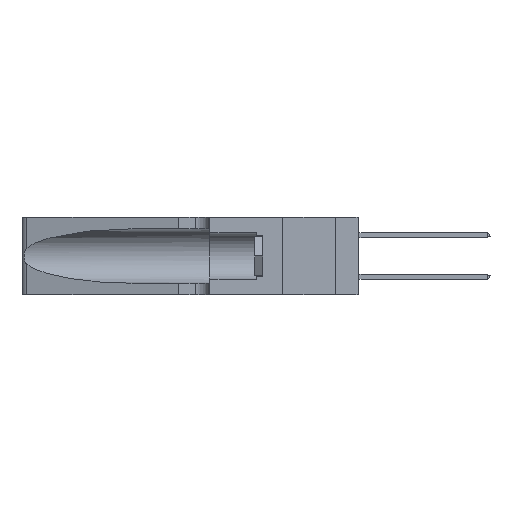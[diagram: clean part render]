
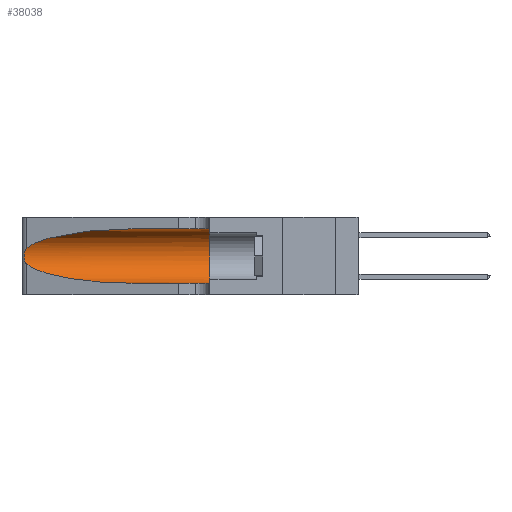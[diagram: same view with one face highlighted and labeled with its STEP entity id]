
A CAD part, left-side view. The second image highlights one B-rep face of the part: STEP entity #38038.
In plain terms, the highlighted cylindrical face has radius 3.308 mm (diameter 6.617 mm), a partial arc.
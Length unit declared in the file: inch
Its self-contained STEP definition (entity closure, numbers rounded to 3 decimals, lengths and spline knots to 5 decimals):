
#648 = CARTESIAN_POINT ( 'NONE',  ( 0.26075, 1.23896, 0.19203 ) ) ;
#742 = CARTESIAN_POINT ( 'NONE',  ( 0.1305, 0.35, 0.185 ) ) ;
#1594 = VERTEX_POINT ( 'NONE', #13156 ) ;
#1955 = VERTEX_POINT ( 'NONE', #30343 ) ;
#3996 = CARTESIAN_POINT ( 'NONE',  ( 0.26017, 1.23833, 0.17102 ) ) ;
#4083 = DIRECTION ( 'NONE',  ( 0., 0., 1. ) ) ;
#4173 = EDGE_CURVE ( 'NONE', #13887, #27170, #16324, .T. ) ;
#4874 = CARTESIAN_POINT ( 'NONE',  ( 0.2373, 1.15595, 0.08982 ) ) ;
#6725 = EDGE_CURVE ( 'NONE', #24752, #1955, #17842, .T. ) ;
#7201 = CARTESIAN_POINT ( 'NONE',  ( 0.25789, 1.23486, 0.15765 ) ) ;
#7858 = EDGE_CURVE ( 'NONE', #10722, #27170, #9603, .T. ) ;
#7879 = VECTOR ( 'NONE', #23334, 39.37008 ) ;
#7884 = ORIENTED_EDGE ( 'NONE', *, *, #4173, .T. ) ;
#9211 = CARTESIAN_POINT ( 'NONE',  ( 0.1305, 0.35, 0.31525 ) ) ;
#9603 = CIRCLE ( 'NONE', #31955, 0.13025 ) ;
#10270 = CARTESIAN_POINT ( 'NONE',  ( 0.25555, 1.22994, 0.2215 ) ) ;
#10422 = CARTESIAN_POINT ( 'NONE',  ( 0.25555, 1.22993, 0.14849 ) ) ;
#10722 = VERTEX_POINT ( 'NONE', #9211 ) ;
#11773 = VECTOR ( 'NONE', #40922, 39.37008 ) ;
#11807 = ORIENTED_EDGE ( 'NONE', *, *, #6725, .T. ) ;
#11838 = CARTESIAN_POINT ( 'NONE',  ( 0.1305, 0.72297, 0.31525 ) ) ;
#12686 = CARTESIAN_POINT ( 'NONE',  ( 0.1305, 1.61858, 0.31525 ) ) ;
#13156 = CARTESIAN_POINT ( 'NONE',  ( 0.25487, 1.22718, 0.14631 ) ) ;
#13887 = VERTEX_POINT ( 'NONE', #14774 ) ;
#14275 = EDGE_CURVE ( 'NONE', #1955, #1594, #14800, .T. ) ;
#14774 = CARTESIAN_POINT ( 'NONE',  ( 0.1305, 0.72297, 0.05475 ) ) ;
#14800 = B_SPLINE_CURVE_WITH_KNOTS ( 'NONE', 3,
 ( #26027, #10270, #35518, #16672, #38685, #19842, #648, #23006, #3996, #26154, #7201, #29315, #10422, #32488 ),
 .UNSPECIFIED., .F., .F.,
 ( 4, 2, 2, 2, 2, 2, 4 ),
 ( 0., 0.00027, 0.00053, 0.00107, 0.0016, 0.00187, 0.00214 ),
 .UNSPECIFIED. ) ;
#15028 = CARTESIAN_POINT ( 'NONE',  ( 0.2373, 1.15595, 0.28018 ) ) ;
#15487 = ORIENTED_EDGE ( 'NONE', *, *, #14275, .T. ) ;
#16324 = LINE ( 'NONE', #17003, #7879 ) ;
#16672 = CARTESIAN_POINT ( 'NONE',  ( 0.25787, 1.23484, 0.2124 ) ) ;
#17003 = CARTESIAN_POINT ( 'NONE',  ( 0.1305, 1.61858, 0.05475 ) ) ;
#17670 = CARTESIAN_POINT ( 'NONE',  ( 0.1305, 1.61858, 0.185 ) ) ;
#17842 =( BOUNDED_CURVE ( )  B_SPLINE_CURVE ( 3, ( #11838, #18088, #15028, #37061 ),
 .UNSPECIFIED., .F., .T. ) 
 B_SPLINE_CURVE_WITH_KNOTS ( ( 4, 4 ),
 ( 1.5708, 2.84003 ),
 .UNSPECIFIED. ) 
 CURVE ( )  GEOMETRIC_REPRESENTATION_ITEM ( )  RATIONAL_B_SPLINE_CURVE ( ( 1., 0.87, 0.87, 1. ) ) 
 REPRESENTATION_ITEM ( '' )  );
#18088 = CARTESIAN_POINT ( 'NONE',  ( 0.18966, 0.96281, 0.31525 ) ) ;
#18722 = ORIENTED_EDGE ( 'NONE', *, *, #7858, .F. ) ;
#19085 =( BOUNDED_CURVE ( )  B_SPLINE_CURVE ( 3, ( #33361, #4874, #39678, #20843 ),
 .UNSPECIFIED., .F., .T. ) 
 B_SPLINE_CURVE_WITH_KNOTS ( ( 4, 4 ),
 ( 3.44316, 4.71239 ),
 .UNSPECIFIED. ) 
 CURVE ( )  GEOMETRIC_REPRESENTATION_ITEM ( )  RATIONAL_B_SPLINE_CURVE ( ( 1., 0.87, 0.87, 1. ) ) 
 REPRESENTATION_ITEM ( '' )  );
#19842 = CARTESIAN_POINT ( 'NONE',  ( 0.26018, 1.23835, 0.19895 ) ) ;
#20843 = CARTESIAN_POINT ( 'NONE',  ( 0.1305, 0.72297, 0.05475 ) ) ;
#21169 = LINE ( 'NONE', #12686, #11773 ) ;
#23006 = CARTESIAN_POINT ( 'NONE',  ( 0.26075, 1.23896, 0.178 ) ) ;
#23086 = DIRECTION ( 'NONE',  ( 0., 1., 0. ) ) ;
#23334 = DIRECTION ( 'NONE',  ( 0., -1., 0. ) ) ;
#23385 = FACE_OUTER_BOUND ( 'NONE', #35616, .T. ) ;
#24012 = DIRECTION ( 'NONE',  ( 0., -1., 0. ) ) ;
#24699 = EDGE_CURVE ( 'NONE', #24752, #10722, #21169, .T. ) ;
#24752 = VERTEX_POINT ( 'NONE', #28782 ) ;
#26027 = CARTESIAN_POINT ( 'NONE',  ( 0.25487, 1.22718, 0.22369 ) ) ;
#26154 = CARTESIAN_POINT ( 'NONE',  ( 0.25856, 1.23593, 0.16098 ) ) ;
#27170 = VERTEX_POINT ( 'NONE', #35934 ) ;
#27775 = ORIENTED_EDGE ( 'NONE', *, *, #28584, .T. ) ;
#28584 = EDGE_CURVE ( 'NONE', #1594, #13887, #19085, .T. ) ;
#28782 = CARTESIAN_POINT ( 'NONE',  ( 0.1305, 0.72297, 0.31525 ) ) ;
#29315 = CARTESIAN_POINT ( 'NONE',  ( 0.25639, 1.23186, 0.15144 ) ) ;
#30343 = CARTESIAN_POINT ( 'NONE',  ( 0.25487, 1.22718, 0.22369 ) ) ;
#30751 = CYLINDRICAL_SURFACE ( 'NONE', #32991, 0.13025 ) ;
#31955 = AXIS2_PLACEMENT_3D ( 'NONE', #742, #23086, #4083 ) ;
#32488 = CARTESIAN_POINT ( 'NONE',  ( 0.25487, 1.22718, 0.14631 ) ) ;
#32991 = AXIS2_PLACEMENT_3D ( 'NONE', #17670, #24012, #36531 ) ;
#33361 = CARTESIAN_POINT ( 'NONE',  ( 0.25487, 1.22718, 0.14631 ) ) ;
#33546 = ORIENTED_EDGE ( 'NONE', *, *, #24699, .F. ) ;
#35518 = CARTESIAN_POINT ( 'NONE',  ( 0.25639, 1.23184, 0.21858 ) ) ;
#35616 = EDGE_LOOP ( 'NONE', ( #11807, #15487, #27775, #7884, #18722, #33546 ) ) ;
#35934 = CARTESIAN_POINT ( 'NONE',  ( 0.1305, 0.35, 0.05475 ) ) ;
#36531 = DIRECTION ( 'NONE',  ( 0., 0., -1. ) ) ;
#37061 = CARTESIAN_POINT ( 'NONE',  ( 0.25487, 1.22718, 0.22369 ) ) ;
#38038 = ADVANCED_FACE ( 'NONE', ( #23385 ), #30751, .F. ) ;
#38685 = CARTESIAN_POINT ( 'NONE',  ( 0.25854, 1.2359, 0.20912 ) ) ;
#39678 = CARTESIAN_POINT ( 'NONE',  ( 0.18966, 0.96281, 0.05475 ) ) ;
#40922 = DIRECTION ( 'NONE',  ( 0., -1., 0. ) ) ;
